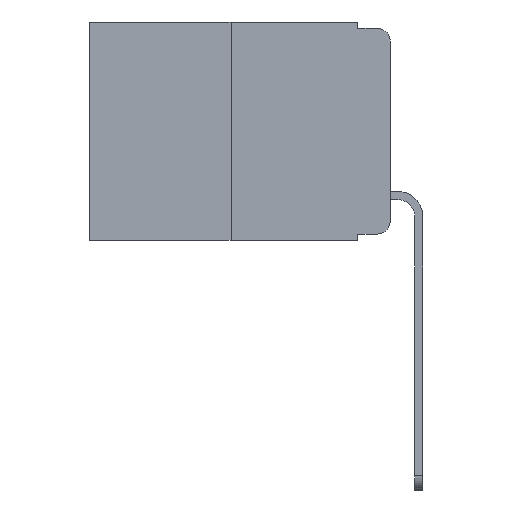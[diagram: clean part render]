
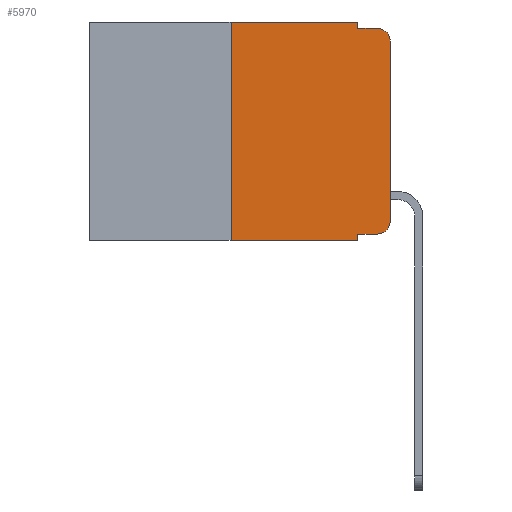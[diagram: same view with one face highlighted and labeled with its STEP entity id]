
A CAD part, left-side view. The second image highlights one B-rep face of the part: STEP entity #5970.
In plain terms, the highlighted planar face has unit normal (-1, 0, 0).
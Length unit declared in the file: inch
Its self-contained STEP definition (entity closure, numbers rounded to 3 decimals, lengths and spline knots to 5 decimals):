
#140 = VECTOR ( 'NONE', #3971, 39.37008 ) ;
#469 = VERTEX_POINT ( 'NONE', #6618 ) ;
#664 = EDGE_LOOP ( 'NONE', ( #1125, #5033, #8360, #4866, #8205, #4284, #3379, #6722, #790, #2511 ) ) ;
#689 = DIRECTION ( 'NONE',  ( 0., 0., -1. ) ) ;
#775 = AXIS2_PLACEMENT_3D ( 'NONE', #11607, #6382, #689 ) ;
#790 = ORIENTED_EDGE ( 'NONE', *, *, #6613, .T. ) ;
#863 = CARTESIAN_POINT ( 'NONE',  ( 0., 0.25, 0. ) ) ;
#945 = DIRECTION ( 'NONE',  ( -1., 0., 0. ) ) ;
#1125 = ORIENTED_EDGE ( 'NONE', *, *, #10012, .T. ) ;
#1443 = VERTEX_POINT ( 'NONE', #5634 ) ;
#1496 = CARTESIAN_POINT ( 'NONE',  ( 0., 0.051, 0. ) ) ;
#1969 = CARTESIAN_POINT ( 'NONE',  ( 0., 0.051, -0.333 ) ) ;
#1985 = VECTOR ( 'NONE', #11674, 39.37008 ) ;
#2102 = LINE ( 'NONE', #1496, #9085 ) ;
#2251 = VECTOR ( 'NONE', #10030, 39.37008 ) ;
#2511 = ORIENTED_EDGE ( 'NONE', *, *, #10923, .T. ) ;
#2697 = DIRECTION ( 'NONE',  ( 0., -1., 0. ) ) ;
#3066 = CIRCLE ( 'NONE', #775, 0.02 ) ;
#3125 = VERTEX_POINT ( 'NONE', #8890 ) ;
#3379 = ORIENTED_EDGE ( 'NONE', *, *, #5639, .T. ) ;
#3697 = VERTEX_POINT ( 'NONE', #6270 ) ;
#3746 = CIRCLE ( 'NONE', #9006, 0.02 ) ;
#3824 = DIRECTION ( 'NONE',  ( 0., 0., 1. ) ) ;
#3971 = DIRECTION ( 'NONE',  ( 0., -1., 0. ) ) ;
#4284 = ORIENTED_EDGE ( 'NONE', *, *, #4506, .F. ) ;
#4319 = LINE ( 'NONE', #1969, #6448 ) ;
#4506 = EDGE_CURVE ( 'NONE', #5767, #10692, #10477, .T. ) ;
#4713 = CARTESIAN_POINT ( 'NONE',  ( 0., 0., 0. ) ) ;
#4866 = ORIENTED_EDGE ( 'NONE', *, *, #9860, .F. ) ;
#5033 = ORIENTED_EDGE ( 'NONE', *, *, #8250, .T. ) ;
#5090 = LINE ( 'NONE', #4713, #2251 ) ;
#5227 = VERTEX_POINT ( 'NONE', #11295 ) ;
#5345 = LINE ( 'NONE', #6698, #140 ) ;
#5558 = CARTESIAN_POINT ( 'NONE',  ( 0., 0.051, 0. ) ) ;
#5634 = CARTESIAN_POINT ( 'NONE',  ( 0., 0.051, -0.333 ) ) ;
#5639 = EDGE_CURVE ( 'NONE', #5767, #8799, #11661, .T. ) ;
#5767 = VERTEX_POINT ( 'NONE', #8910 ) ;
#5970 = ADVANCED_FACE ( 'NONE', ( #11241 ), #11871, .F. ) ;
#6082 = CARTESIAN_POINT ( 'NONE',  ( 0., 0.25, 0. ) ) ;
#6270 = CARTESIAN_POINT ( 'NONE',  ( 0., 0.051, 0. ) ) ;
#6382 = DIRECTION ( 'NONE',  ( -1., 0., 0. ) ) ;
#6448 = VECTOR ( 'NONE', #10581, 39.37008 ) ;
#6613 = EDGE_CURVE ( 'NONE', #1443, #10431, #4319, .T. ) ;
#6618 = CARTESIAN_POINT ( 'NONE',  ( 0., 0., -0.313 ) ) ;
#6619 = CARTESIAN_POINT ( 'NONE',  ( 0., 0.02, -0.313 ) ) ;
#6698 = CARTESIAN_POINT ( 'NONE',  ( 0., 0.051, -0.01 ) ) ;
#6722 = ORIENTED_EDGE ( 'NONE', *, *, #8936, .F. ) ;
#7043 = VECTOR ( 'NONE', #2697, 39.37008 ) ;
#7137 = CARTESIAN_POINT ( 'NONE',  ( 0., 0.051, -0.343 ) ) ;
#7314 = LINE ( 'NONE', #7332, #7043 ) ;
#7332 = CARTESIAN_POINT ( 'NONE',  ( 0., 0.473, 0. ) ) ;
#7358 = CARTESIAN_POINT ( 'NONE',  ( 0., 0.473, -0.343 ) ) ;
#7454 = CARTESIAN_POINT ( 'NONE',  ( 0., 0.02, -0.333 ) ) ;
#7517 = DIRECTION ( 'NONE',  ( 0., 0., -1. ) ) ;
#8083 = DIRECTION ( 'NONE',  ( 0., -1., 0. ) ) ;
#8139 = VECTOR ( 'NONE', #3824, 39.37008 ) ;
#8205 = ORIENTED_EDGE ( 'NONE', *, *, #10846, .F. ) ;
#8250 = EDGE_CURVE ( 'NONE', #5227, #10983, #3066, .T. ) ;
#8360 = ORIENTED_EDGE ( 'NONE', *, *, #11019, .F. ) ;
#8799 = VERTEX_POINT ( 'NONE', #7137 ) ;
#8890 = CARTESIAN_POINT ( 'NONE',  ( 0., 0.051, -0.01 ) ) ;
#8910 = CARTESIAN_POINT ( 'NONE',  ( 0., 0.25, -0.343 ) ) ;
#8936 = EDGE_CURVE ( 'NONE', #1443, #8799, #11836, .T. ) ;
#9006 = AXIS2_PLACEMENT_3D ( 'NONE', #6619, #945, #7517 ) ;
#9085 = VECTOR ( 'NONE', #9758, 39.37008 ) ;
#9278 = CARTESIAN_POINT ( 'NONE',  ( 0., 0.02, -0.01 ) ) ;
#9341 = VECTOR ( 'NONE', #8083, 39.37008 ) ;
#9758 = DIRECTION ( 'NONE',  ( 0., 0., -1. ) ) ;
#9860 = EDGE_CURVE ( 'NONE', #3697, #3125, #2102, .T. ) ;
#10012 = EDGE_CURVE ( 'NONE', #469, #5227, #5090, .T. ) ;
#10030 = DIRECTION ( 'NONE',  ( 0., 0., 1. ) ) ;
#10384 = AXIS2_PLACEMENT_3D ( 'NONE', #11432, #11396, #11897 ) ;
#10431 = VERTEX_POINT ( 'NONE', #7454 ) ;
#10477 = LINE ( 'NONE', #863, #8139 ) ;
#10581 = DIRECTION ( 'NONE',  ( 0., -1., 0. ) ) ;
#10692 = VERTEX_POINT ( 'NONE', #6082 ) ;
#10846 = EDGE_CURVE ( 'NONE', #10692, #3697, #7314, .T. ) ;
#10923 = EDGE_CURVE ( 'NONE', #10431, #469, #3746, .T. ) ;
#10983 = VERTEX_POINT ( 'NONE', #9278 ) ;
#11019 = EDGE_CURVE ( 'NONE', #3125, #10983, #5345, .T. ) ;
#11241 = FACE_OUTER_BOUND ( 'NONE', #664, .T. ) ;
#11295 = CARTESIAN_POINT ( 'NONE',  ( 0., 0., -0.03 ) ) ;
#11396 = DIRECTION ( 'NONE',  ( 1., 0., 0. ) ) ;
#11432 = CARTESIAN_POINT ( 'NONE',  ( 0., 0.473, 0. ) ) ;
#11607 = CARTESIAN_POINT ( 'NONE',  ( 0., 0.02, -0.03 ) ) ;
#11661 = LINE ( 'NONE', #7358, #9341 ) ;
#11674 = DIRECTION ( 'NONE',  ( 0., 0., -1. ) ) ;
#11836 = LINE ( 'NONE', #5558, #1985 ) ;
#11871 = PLANE ( 'NONE',  #10384 ) ;
#11897 = DIRECTION ( 'NONE',  ( 0., 0., -1. ) ) ;
